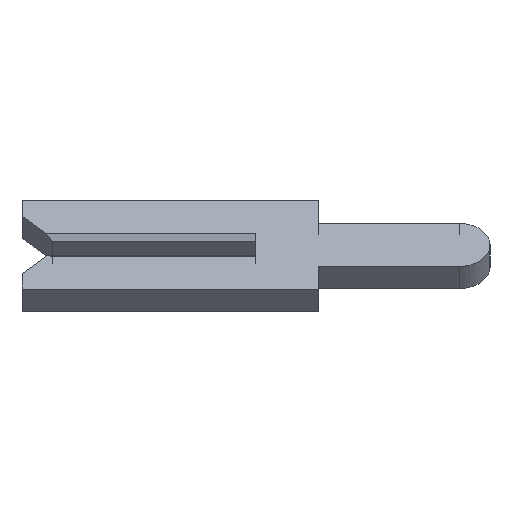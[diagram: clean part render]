
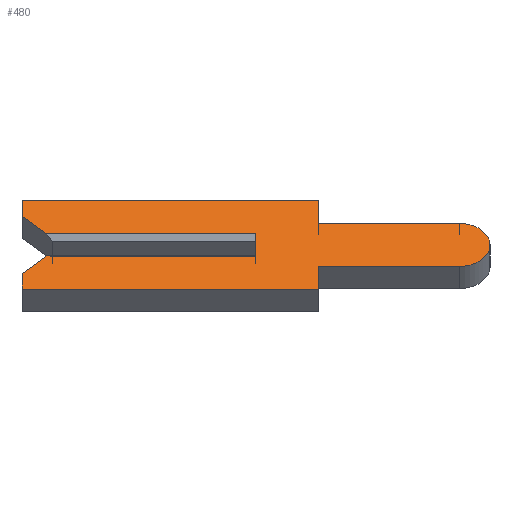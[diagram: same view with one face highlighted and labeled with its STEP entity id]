
A CAD part, left-side view. The second image highlights one B-rep face of the part: STEP entity #480.
In plain terms, the highlighted face is planar.
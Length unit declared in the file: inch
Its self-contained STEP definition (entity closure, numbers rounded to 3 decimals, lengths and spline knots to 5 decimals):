
#6 = DIRECTION ( 'NONE',  ( 0., -0.707, 0.707 ) ) ;
#12 = VECTOR ( 'NONE', #1023, 39.37008 ) ;
#13 = DIRECTION ( 'NONE',  ( 0., 0., 1. ) ) ;
#67 = EDGE_CURVE ( 'NONE', #1903, #1479, #1367, .T. ) ;
#98 = VECTOR ( 'NONE', #1882, 39.37008 ) ;
#113 = CARTESIAN_POINT ( 'NONE',  ( -0.01, -0.1305, -0.0195 ) ) ;
#157 = VECTOR ( 'NONE', #6, 39.37008 ) ;
#161 = CARTESIAN_POINT ( 'NONE',  ( -0.01, -0.1305, -0.01 ) ) ;
#167 = CARTESIAN_POINT ( 'NONE',  ( -0.01, 0.15, 0.04 ) ) ;
#170 = VERTEX_POINT ( 'NONE', #331 ) ;
#172 = VERTEX_POINT ( 'NONE', #506 ) ;
#209 = DIRECTION ( 'NONE',  ( 0., 0.707, 0.707 ) ) ;
#220 = CARTESIAN_POINT ( 'NONE',  ( -0.01, -0.04, -0.04 ) ) ;
#230 = CARTESIAN_POINT ( 'NONE',  ( -0.01, 0.15, 0.026 ) ) ;
#258 = DIRECTION ( 'NONE',  ( 0., 0., 1. ) ) ;
#271 = DIRECTION ( 'NONE',  ( 1., 0., 0. ) ) ;
#282 = VERTEX_POINT ( 'NONE', #944 ) ;
#296 = LINE ( 'NONE', #1975, #12 ) ;
#298 = VECTOR ( 'NONE', #589, 39.37008 ) ;
#320 = EDGE_CURVE ( 'NONE', #1844, #1394, #1446, .T. ) ;
#331 = CARTESIAN_POINT ( 'NONE',  ( -0.01, 0.134, -0.01 ) ) ;
#345 = CARTESIAN_POINT ( 'NONE',  ( -0.01, -0.1305, 0. ) ) ;
#368 = EDGE_CURVE ( 'NONE', #1726, #282, #729, .T. ) ;
#393 = DIRECTION ( 'NONE',  ( 0., 0., 1. ) ) ;
#423 = LINE ( 'NONE', #220, #1658 ) ;
#443 = AXIS2_PLACEMENT_3D ( 'NONE', #345, #667, #951 ) ;
#462 = CARTESIAN_POINT ( 'NONE',  ( -0.01, -0.04, 0.04 ) ) ;
#473 = CARTESIAN_POINT ( 'NONE',  ( -0.01, 0.134, 0.01 ) ) ;
#480 = ADVANCED_FACE ( 'NONE', ( #1183 ), #802, .F. ) ;
#483 = VERTEX_POINT ( 'NONE', #1747 ) ;
#495 = CARTESIAN_POINT ( 'NONE',  ( -0.01, -0.04, -0.0195 ) ) ;
#506 = CARTESIAN_POINT ( 'NONE',  ( -0.01, -0.04, -0.04 ) ) ;
#537 = VERTEX_POINT ( 'NONE', #495 ) ;
#589 = DIRECTION ( 'NONE',  ( 0., 1., 0. ) ) ;
#611 = EDGE_CURVE ( 'NONE', #537, #172, #423, .T. ) ;
#614 = LINE ( 'NONE', #1527, #157 ) ;
#620 = VECTOR ( 'NONE', #1576, 39.37008 ) ;
#667 = DIRECTION ( 'NONE',  ( 1., 0., 0. ) ) ;
#729 = LINE ( 'NONE', #1916, #1151 ) ;
#766 = ORIENTED_EDGE ( 'NONE', *, *, #1187, .F. ) ;
#790 = VECTOR ( 'NONE', #1235, 39.37008 ) ;
#802 = PLANE ( 'NONE',  #443 ) ;
#862 = ORIENTED_EDGE ( 'NONE', *, *, #1786, .F. ) ;
#870 = ORIENTED_EDGE ( 'NONE', *, *, #611, .F. ) ;
#892 = CARTESIAN_POINT ( 'NONE',  ( -0.01, 0., 0.0065 ) ) ;
#898 = LINE ( 'NONE', #1766, #920 ) ;
#905 = ORIENTED_EDGE ( 'NONE', *, *, #1021, .F. ) ;
#908 = CARTESIAN_POINT ( 'NONE',  ( -0.01, -0.04, 0.04 ) ) ;
#920 = VECTOR ( 'NONE', #1802, 39.37008 ) ;
#923 = CARTESIAN_POINT ( 'NONE',  ( -0.01, 0.15, -0.026 ) ) ;
#944 = CARTESIAN_POINT ( 'NONE',  ( -0.01, 0.15, 0.026 ) ) ;
#951 = DIRECTION ( 'NONE',  ( 0., 0., -1. ) ) ;
#985 = ORIENTED_EDGE ( 'NONE', *, *, #1115, .F. ) ;
#993 = VECTOR ( 'NONE', #393, 39.37008 ) ;
#1014 = ORIENTED_EDGE ( 'NONE', *, *, #1642, .F. ) ;
#1016 = DIRECTION ( 'NONE',  ( 0., 0., -1. ) ) ;
#1021 = EDGE_CURVE ( 'NONE', #282, #1903, #1834, .T. ) ;
#1023 = DIRECTION ( 'NONE',  ( 0., -1., 0. ) ) ;
#1028 = ORIENTED_EDGE ( 'NONE', *, *, #1712, .F. ) ;
#1045 = DIRECTION ( 'NONE',  ( 0., 0., -1. ) ) ;
#1084 = LINE ( 'NONE', #923, #1873 ) ;
#1086 = ORIENTED_EDGE ( 'NONE', *, *, #320, .F. ) ;
#1115 = EDGE_CURVE ( 'NONE', #1153, #537, #898, .T. ) ;
#1117 = LINE ( 'NONE', #1674, #298 ) ;
#1151 = VECTOR ( 'NONE', #209, 39.37008 ) ;
#1153 = VERTEX_POINT ( 'NONE', #113 ) ;
#1173 = CARTESIAN_POINT ( 'NONE',  ( -0.01, -0.1305, 0. ) ) ;
#1183 = FACE_OUTER_BOUND ( 'NONE', #1569, .T. ) ;
#1187 = EDGE_CURVE ( 'NONE', #1394, #1153, #1783, .T. ) ;
#1235 = DIRECTION ( 'NONE',  ( 0., -1., 0. ) ) ;
#1248 = ORIENTED_EDGE ( 'NONE', *, *, #1319, .F. ) ;
#1267 = EDGE_CURVE ( 'NONE', #172, #1284, #1117, .T. ) ;
#1284 = VERTEX_POINT ( 'NONE', #1663 ) ;
#1296 = ORIENTED_EDGE ( 'NONE', *, *, #368, .F. ) ;
#1319 = EDGE_CURVE ( 'NONE', #1624, #483, #1862, .T. ) ;
#1331 = ORIENTED_EDGE ( 'NONE', *, *, #1401, .T. ) ;
#1335 = ORIENTED_EDGE ( 'NONE', *, *, #67, .F. ) ;
#1367 = LINE ( 'NONE', #1551, #98 ) ;
#1386 = CARTESIAN_POINT ( 'NONE',  ( -0.01, -0.04, 0.0195 ) ) ;
#1394 = VERTEX_POINT ( 'NONE', #1655 ) ;
#1396 = LINE ( 'NONE', #161, #790 ) ;
#1401 = EDGE_CURVE ( 'NONE', #1726, #483, #296, .T. ) ;
#1419 = DIRECTION ( 'NONE',  ( 0., 0., -1. ) ) ;
#1432 = VERTEX_POINT ( 'NONE', #1542 ) ;
#1434 = CARTESIAN_POINT ( 'NONE',  ( -0.01, -0.04, 0.0195 ) ) ;
#1446 = LINE ( 'NONE', #1434, #620 ) ;
#1454 = VECTOR ( 'NONE', #1419, 39.37008 ) ;
#1479 = VERTEX_POINT ( 'NONE', #462 ) ;
#1527 = CARTESIAN_POINT ( 'NONE',  ( -0.01, 0.1305, -0.0065 ) ) ;
#1542 = CARTESIAN_POINT ( 'NONE',  ( -0.01, 0.15, -0.026 ) ) ;
#1551 = CARTESIAN_POINT ( 'NONE',  ( -0.01, 0.15, 0.04 ) ) ;
#1569 = EDGE_LOOP ( 'NONE', ( #1331, #1248, #862, #1014, #1815, #1749, #870, #985, #766, #1086, #1028, #1335, #905, #1296 ) ) ;
#1576 = DIRECTION ( 'NONE',  ( 0., -1., 0. ) ) ;
#1624 = VERTEX_POINT ( 'NONE', #1863 ) ;
#1642 = EDGE_CURVE ( 'NONE', #1432, #170, #614, .T. ) ;
#1655 = CARTESIAN_POINT ( 'NONE',  ( -0.01, -0.1305, 0.0195 ) ) ;
#1658 = VECTOR ( 'NONE', #1016, 39.37008 ) ;
#1663 = CARTESIAN_POINT ( 'NONE',  ( -0.01, 0.15, -0.04 ) ) ;
#1674 = CARTESIAN_POINT ( 'NONE',  ( -0.01, 0.15, -0.04 ) ) ;
#1712 = EDGE_CURVE ( 'NONE', #1479, #1844, #1978, .T. ) ;
#1726 = VERTEX_POINT ( 'NONE', #473 ) ;
#1747 = CARTESIAN_POINT ( 'NONE',  ( -0.01, 0., 0.01 ) ) ;
#1749 = ORIENTED_EDGE ( 'NONE', *, *, #1267, .F. ) ;
#1766 = CARTESIAN_POINT ( 'NONE',  ( -0.01, -0.04, -0.0195 ) ) ;
#1783 = CIRCLE ( 'NONE', #1858, 0.0195 ) ;
#1786 = EDGE_CURVE ( 'NONE', #170, #1624, #1396, .T. ) ;
#1802 = DIRECTION ( 'NONE',  ( 0., 1., 0. ) ) ;
#1815 = ORIENTED_EDGE ( 'NONE', *, *, #1835, .F. ) ;
#1834 = LINE ( 'NONE', #230, #993 ) ;
#1835 = EDGE_CURVE ( 'NONE', #1284, #1432, #1084, .T. ) ;
#1844 = VERTEX_POINT ( 'NONE', #1386 ) ;
#1858 = AXIS2_PLACEMENT_3D ( 'NONE', #1173, #271, #1045 ) ;
#1862 = LINE ( 'NONE', #892, #1912 ) ;
#1863 = CARTESIAN_POINT ( 'NONE',  ( -0.01, 0., -0.01 ) ) ;
#1873 = VECTOR ( 'NONE', #13, 39.37008 ) ;
#1882 = DIRECTION ( 'NONE',  ( 0., -1., 0. ) ) ;
#1903 = VERTEX_POINT ( 'NONE', #167 ) ;
#1912 = VECTOR ( 'NONE', #258, 39.37008 ) ;
#1916 = CARTESIAN_POINT ( 'NONE',  ( -0.01, 0.1305, 0.0065 ) ) ;
#1975 = CARTESIAN_POINT ( 'NONE',  ( -0.01, 0.15, 0.01 ) ) ;
#1978 = LINE ( 'NONE', #908, #1454 ) ;
